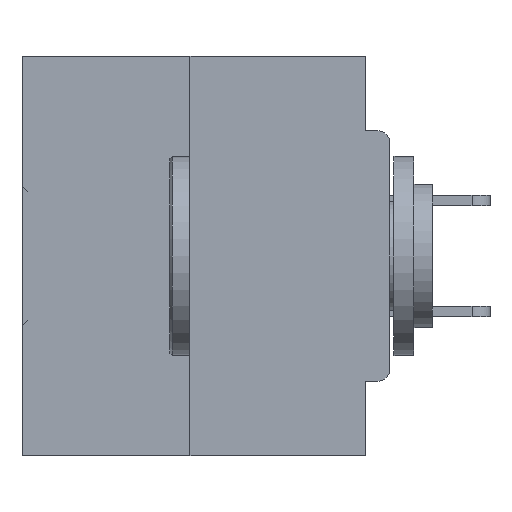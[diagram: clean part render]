
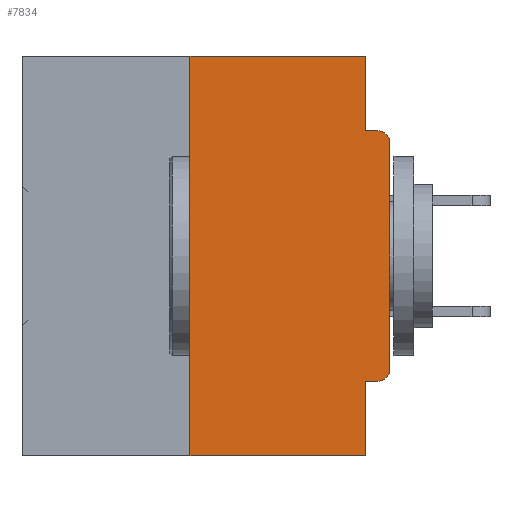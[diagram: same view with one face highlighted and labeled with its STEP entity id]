
A CAD part, left-side view. The second image highlights one B-rep face of the part: STEP entity #7834.
In plain terms, the highlighted planar face has unit normal (-1, 0, 0).
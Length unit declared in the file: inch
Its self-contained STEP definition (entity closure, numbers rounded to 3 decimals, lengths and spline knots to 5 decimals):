
#315 = VECTOR ( 'NONE', #21365, 39.37008 ) ;
#384 = ORIENTED_EDGE ( 'NONE', *, *, #25298, .F. ) ;
#646 = LINE ( 'NONE', #8451, #18354 ) ;
#1198 = EDGE_CURVE ( 'NONE', #41330, #19763, #31895, .T. ) ;
#1292 = DIRECTION ( 'NONE',  ( -1., 0., 0. ) ) ;
#1592 = VECTOR ( 'NONE', #9251, 39.37008 ) ;
#1762 = DIRECTION ( 'NONE',  ( 0., 0., -1. ) ) ;
#2135 = CARTESIAN_POINT ( 'NONE',  ( 0., 0.031, 0. ) ) ;
#2511 = EDGE_CURVE ( 'NONE', #15376, #32339, #4978, .T. ) ;
#3367 = CARTESIAN_POINT ( 'NONE',  ( 0., 0.015, -0.4065 ) ) ;
#4828 = VECTOR ( 'NONE', #17786, 39.37008 ) ;
#4978 = LINE ( 'NONE', #39589, #44478 ) ;
#5807 = DIRECTION ( 'NONE',  ( -1., 0., 0. ) ) ;
#6579 = VERTEX_POINT ( 'NONE', #2135 ) ;
#6859 = AXIS2_PLACEMENT_3D ( 'NONE', #27670, #5807, #31328 ) ;
#7834 = ADVANCED_FACE ( 'NONE', ( #9647 ), #12896, .F. ) ;
#7891 = EDGE_LOOP ( 'NONE', ( #27754, #40033, #21297, #19263, #22572, #23693, #45441, #32077, #384, #28908 ) ) ;
#8451 = CARTESIAN_POINT ( 'NONE',  ( 0., 0., -0.0935 ) ) ;
#9251 = DIRECTION ( 'NONE',  ( 0., 0., 1. ) ) ;
#9588 = EDGE_CURVE ( 'NONE', #42475, #30466, #35170, .T. ) ;
#9647 = FACE_OUTER_BOUND ( 'NONE', #7891, .T. ) ;
#10909 = CARTESIAN_POINT ( 'NONE',  ( 0., 0.25, 0. ) ) ;
#11031 = EDGE_CURVE ( 'NONE', #42475, #41330, #46471, .T. ) ;
#11145 = VERTEX_POINT ( 'NONE', #26268 ) ;
#12896 = PLANE ( 'NONE',  #26675 ) ;
#13037 = AXIS2_PLACEMENT_3D ( 'NONE', #42274, #1292, #1762 ) ;
#15376 = VERTEX_POINT ( 'NONE', #27558 ) ;
#16099 = CARTESIAN_POINT ( 'NONE',  ( 0., 0., 0. ) ) ;
#17786 = DIRECTION ( 'NONE',  ( 0., 1., 0. ) ) ;
#18354 = VECTOR ( 'NONE', #30441, 39.37008 ) ;
#18387 = LINE ( 'NONE', #46178, #32079 ) ;
#19263 = ORIENTED_EDGE ( 'NONE', *, *, #33532, .F. ) ;
#19763 = VERTEX_POINT ( 'NONE', #32341 ) ;
#20702 = DIRECTION ( 'NONE',  ( 0., 0., -1. ) ) ;
#21297 = ORIENTED_EDGE ( 'NONE', *, *, #2511, .T. ) ;
#21365 = DIRECTION ( 'NONE',  ( 0., 0., 1. ) ) ;
#21949 = EDGE_CURVE ( 'NONE', #15376, #39781, #23187, .T. ) ;
#22572 = ORIENTED_EDGE ( 'NONE', *, *, #9588, .F. ) ;
#22722 = DIRECTION ( 'NONE',  ( 0., -1., 0. ) ) ;
#23187 = LINE ( 'NONE', #28556, #315 ) ;
#23693 = ORIENTED_EDGE ( 'NONE', *, *, #11031, .T. ) ;
#24823 = VERTEX_POINT ( 'NONE', #31087 ) ;
#25298 = EDGE_CURVE ( 'NONE', #11145, #24823, #646, .T. ) ;
#26268 = CARTESIAN_POINT ( 'NONE',  ( 0., 0.031, -0.0935 ) ) ;
#26675 = AXIS2_PLACEMENT_3D ( 'NONE', #27605, #42376, #46027 ) ;
#27558 = CARTESIAN_POINT ( 'NONE',  ( 0., 0.25, -0.5 ) ) ;
#27566 = VECTOR ( 'NONE', #31919, 39.37008 ) ;
#27605 = CARTESIAN_POINT ( 'NONE',  ( 0., 0.46, 0. ) ) ;
#27670 = CARTESIAN_POINT ( 'NONE',  ( 0., 0.015, -0.1085 ) ) ;
#27754 = ORIENTED_EDGE ( 'NONE', *, *, #39840, .F. ) ;
#28556 = CARTESIAN_POINT ( 'NONE',  ( 0., 0.25, 0. ) ) ;
#28652 = DIRECTION ( 'NONE',  ( 0., -1., 0. ) ) ;
#28908 = ORIENTED_EDGE ( 'NONE', *, *, #38392, .F. ) ;
#28945 = CARTESIAN_POINT ( 'NONE',  ( 0., 0., -0.4065 ) ) ;
#30441 = DIRECTION ( 'NONE',  ( 0., -1., 0. ) ) ;
#30466 = VERTEX_POINT ( 'NONE', #42568 ) ;
#31087 = CARTESIAN_POINT ( 'NONE',  ( 0., 0.015, -0.0935 ) ) ;
#31328 = DIRECTION ( 'NONE',  ( 0., 0., -1. ) ) ;
#31895 = LINE ( 'NONE', #16099, #1592 ) ;
#31919 = DIRECTION ( 'NONE',  ( 0., 0., -1. ) ) ;
#32077 = ORIENTED_EDGE ( 'NONE', *, *, #36002, .T. ) ;
#32079 = VECTOR ( 'NONE', #20702, 39.37008 ) ;
#32339 = VERTEX_POINT ( 'NONE', #45834 ) ;
#32341 = CARTESIAN_POINT ( 'NONE',  ( 0., 0., -0.1085 ) ) ;
#32551 = CARTESIAN_POINT ( 'NONE',  ( 0., 0., -0.3915 ) ) ;
#33532 = EDGE_CURVE ( 'NONE', #30466, #32339, #18387, .T. ) ;
#35041 = LINE ( 'NONE', #37963, #27566 ) ;
#35170 = LINE ( 'NONE', #28945, #4828 ) ;
#36002 = EDGE_CURVE ( 'NONE', #19763, #24823, #41053, .T. ) ;
#36643 = VECTOR ( 'NONE', #22722, 39.37008 ) ;
#37949 = CARTESIAN_POINT ( 'NONE',  ( 0., 0.46, 0. ) ) ;
#37963 = CARTESIAN_POINT ( 'NONE',  ( 0., 0.031, 0. ) ) ;
#38392 = EDGE_CURVE ( 'NONE', #6579, #11145, #35041, .T. ) ;
#39589 = CARTESIAN_POINT ( 'NONE',  ( 0., 0.46, -0.5 ) ) ;
#39781 = VERTEX_POINT ( 'NONE', #10909 ) ;
#39840 = EDGE_CURVE ( 'NONE', #39781, #6579, #46390, .T. ) ;
#40033 = ORIENTED_EDGE ( 'NONE', *, *, #21949, .F. ) ;
#41053 = CIRCLE ( 'NONE', #6859, 0.015 ) ;
#41330 = VERTEX_POINT ( 'NONE', #32551 ) ;
#42274 = CARTESIAN_POINT ( 'NONE',  ( 0., 0.015, -0.3915 ) ) ;
#42376 = DIRECTION ( 'NONE',  ( 1., 0., 0. ) ) ;
#42475 = VERTEX_POINT ( 'NONE', #3367 ) ;
#42568 = CARTESIAN_POINT ( 'NONE',  ( 0., 0.031, -0.4065 ) ) ;
#44478 = VECTOR ( 'NONE', #28652, 39.37008 ) ;
#45441 = ORIENTED_EDGE ( 'NONE', *, *, #1198, .T. ) ;
#45834 = CARTESIAN_POINT ( 'NONE',  ( 0., 0.031, -0.5 ) ) ;
#46027 = DIRECTION ( 'NONE',  ( 0., 0., -1. ) ) ;
#46178 = CARTESIAN_POINT ( 'NONE',  ( 0., 0.031, -0.5 ) ) ;
#46390 = LINE ( 'NONE', #37949, #36643 ) ;
#46471 = CIRCLE ( 'NONE', #13037, 0.015 ) ;
